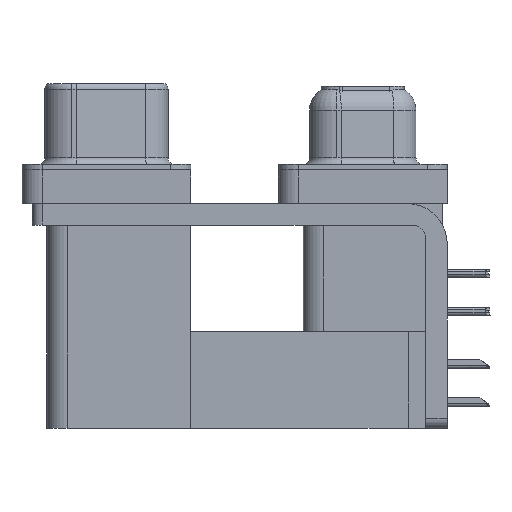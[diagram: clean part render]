
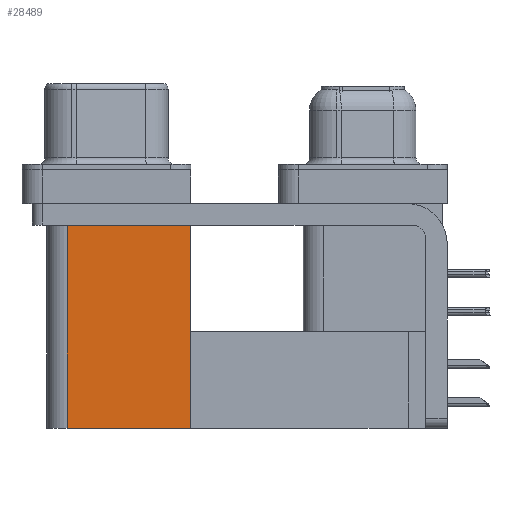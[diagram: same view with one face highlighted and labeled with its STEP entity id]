
A CAD part, left-side view. The second image highlights one B-rep face of the part: STEP entity #28489.
In plain terms, the highlighted planar face has unit normal (-1, 0, 0).
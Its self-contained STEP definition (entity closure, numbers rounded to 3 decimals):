
#902 = LINE ( 'NONE', #13729, #11123 ) ;
#1910 = LINE ( 'NONE', #40186, #7742 ) ;
#3079 = CARTESIAN_POINT ( 'NONE',  ( 3.765, 21.975, -2.5 ) ) ;
#3863 = DIRECTION ( 'NONE',  ( 0., 0., 1. ) ) ;
#5206 = DIRECTION ( 'NONE',  ( 0., 0., 1. ) ) ;
#5618 = CARTESIAN_POINT ( 'NONE',  ( 3.765, 12.775, -19.2 ) ) ;
#7742 = VECTOR ( 'NONE', #11374, 1000. ) ;
#8098 = CARTESIAN_POINT ( 'NONE',  ( 3.765, 12.775, -2.5 ) ) ;
#8104 = ORIENTED_EDGE ( 'NONE', *, *, #22205, .T. ) ;
#8172 = LINE ( 'NONE', #5618, #37428 ) ;
#8756 = PLANE ( 'NONE',  #13501 ) ;
#11123 = VECTOR ( 'NONE', #3863, 1000. ) ;
#11374 = DIRECTION ( 'NONE',  ( 0., 1., 0. ) ) ;
#11447 = DIRECTION ( 'NONE',  ( 0., 1., 0. ) ) ;
#13501 = AXIS2_PLACEMENT_3D ( 'NONE', #21343, #34205, #27883 ) ;
#13714 = VERTEX_POINT ( 'NONE', #27078 ) ;
#13729 = CARTESIAN_POINT ( 'NONE',  ( 3.765, 21.975, -19.2 ) ) ;
#14170 = EDGE_LOOP ( 'NONE', ( #32472, #29306, #15168, #8104 ) ) ;
#15168 = ORIENTED_EDGE ( 'NONE', *, *, #32753, .F. ) ;
#19163 = EDGE_CURVE ( 'NONE', #30094, #20425, #902, .T. ) ;
#19995 = VECTOR ( 'NONE', #11447, 1000. ) ;
#20425 = VERTEX_POINT ( 'NONE', #3079 ) ;
#20831 = CARTESIAN_POINT ( 'NONE',  ( 3.765, 12.775, -19.2 ) ) ;
#21343 = CARTESIAN_POINT ( 'NONE',  ( 3.765, 12.775, -19.2 ) ) ;
#22205 = EDGE_CURVE ( 'NONE', #28082, #13714, #8172, .T. ) ;
#22734 = CARTESIAN_POINT ( 'NONE',  ( 3.765, 21.975, -19.2 ) ) ;
#27078 = CARTESIAN_POINT ( 'NONE',  ( 3.765, 12.775, -2.5 ) ) ;
#27883 = DIRECTION ( 'NONE',  ( 0., 0., -1. ) ) ;
#28082 = VERTEX_POINT ( 'NONE', #20831 ) ;
#28489 = ADVANCED_FACE ( 'NONE', ( #37578 ), #8756, .F. ) ;
#29306 = ORIENTED_EDGE ( 'NONE', *, *, #19163, .F. ) ;
#30094 = VERTEX_POINT ( 'NONE', #22734 ) ;
#30372 = LINE ( 'NONE', #8098, #19995 ) ;
#32472 = ORIENTED_EDGE ( 'NONE', *, *, #37089, .T. ) ;
#32753 = EDGE_CURVE ( 'NONE', #28082, #30094, #1910, .T. ) ;
#34205 = DIRECTION ( 'NONE',  ( 1., 0., 0. ) ) ;
#37089 = EDGE_CURVE ( 'NONE', #13714, #20425, #30372, .T. ) ;
#37428 = VECTOR ( 'NONE', #5206, 1000. ) ;
#37578 = FACE_OUTER_BOUND ( 'NONE', #14170, .T. ) ;
#40186 = CARTESIAN_POINT ( 'NONE',  ( 3.765, 12.775, -19.2 ) ) ;
